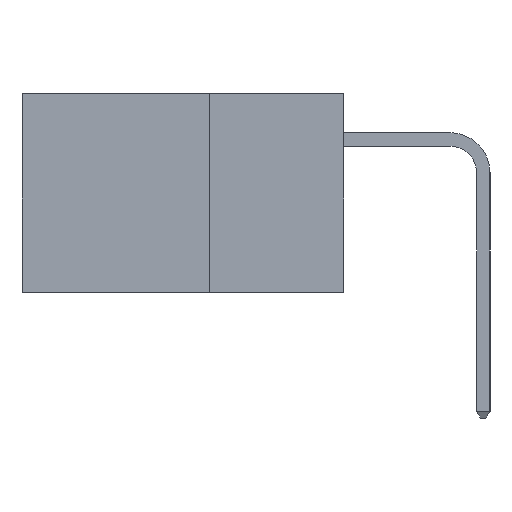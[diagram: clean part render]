
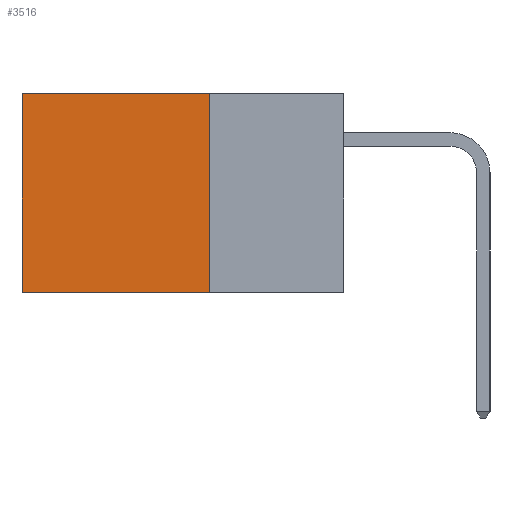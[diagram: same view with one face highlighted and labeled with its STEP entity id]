
A CAD part, left-side view. The second image highlights one B-rep face of the part: STEP entity #3516.
In plain terms, the highlighted planar face has unit normal (-1, 0, 0).
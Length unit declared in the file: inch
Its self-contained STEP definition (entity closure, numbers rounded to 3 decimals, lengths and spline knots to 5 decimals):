
#303 = CARTESIAN_POINT ( 'NONE',  ( 0.298, 0.6, -0.37 ) ) ;
#640 = CARTESIAN_POINT ( 'NONE',  ( 0.298, 0.25, 0. ) ) ;
#1190 = DIRECTION ( 'NONE',  ( 0., 0., -1. ) ) ;
#1357 = VECTOR ( 'NONE', #6439, 39.37008 ) ;
#1404 = VERTEX_POINT ( 'NONE', #2814 ) ;
#2216 = CARTESIAN_POINT ( 'NONE',  ( 0.298, 0.25, -0.37 ) ) ;
#2239 = EDGE_LOOP ( 'NONE', ( #6882, #7178, #5377, #5083 ) ) ;
#2611 = VECTOR ( 'NONE', #7909, 39.37008 ) ;
#2814 = CARTESIAN_POINT ( 'NONE',  ( 0.298, 0.6, 0. ) ) ;
#2846 = EDGE_CURVE ( 'NONE', #8374, #1404, #8167, .T. ) ;
#3516 = ADVANCED_FACE ( 'NONE', ( #6989 ), #6062, .F. ) ;
#3724 = VERTEX_POINT ( 'NONE', #3924 ) ;
#3833 = DIRECTION ( 'NONE',  ( 0., 0., -1. ) ) ;
#3924 = CARTESIAN_POINT ( 'NONE',  ( 0.298, 0.25, -0.37 ) ) ;
#5083 = ORIENTED_EDGE ( 'NONE', *, *, #2846, .T. ) ;
#5377 = ORIENTED_EDGE ( 'NONE', *, *, #9201, .F. ) ;
#5434 = AXIS2_PLACEMENT_3D ( 'NONE', #6059, #9159, #9119 ) ;
#5620 = CARTESIAN_POINT ( 'NONE',  ( 0.298, 0.25, 0. ) ) ;
#6059 = CARTESIAN_POINT ( 'NONE',  ( 0.298, 0.25, 0. ) ) ;
#6062 = PLANE ( 'NONE',  #5434 ) ;
#6166 = EDGE_CURVE ( 'NONE', #3724, #6782, #7071, .T. ) ;
#6439 = DIRECTION ( 'NONE',  ( 0., 1., 0. ) ) ;
#6532 = VECTOR ( 'NONE', #3833, 39.37008 ) ;
#6754 = LINE ( 'NONE', #7030, #6532 ) ;
#6782 = VERTEX_POINT ( 'NONE', #303 ) ;
#6825 = EDGE_CURVE ( 'NONE', #1404, #6782, #6754, .T. ) ;
#6882 = ORIENTED_EDGE ( 'NONE', *, *, #6825, .T. ) ;
#6989 = FACE_OUTER_BOUND ( 'NONE', #2239, .T. ) ;
#7030 = CARTESIAN_POINT ( 'NONE',  ( 0.298, 0.6, 0. ) ) ;
#7071 = LINE ( 'NONE', #2216, #1357 ) ;
#7178 = ORIENTED_EDGE ( 'NONE', *, *, #6166, .F. ) ;
#7909 = DIRECTION ( 'NONE',  ( 0., 1., 0. ) ) ;
#7967 = VECTOR ( 'NONE', #1190, 39.37008 ) ;
#8167 = LINE ( 'NONE', #640, #2611 ) ;
#8172 = LINE ( 'NONE', #5620, #7967 ) ;
#8374 = VERTEX_POINT ( 'NONE', #8658 ) ;
#8658 = CARTESIAN_POINT ( 'NONE',  ( 0.298, 0.25, 0. ) ) ;
#9119 = DIRECTION ( 'NONE',  ( 0., 0., -1. ) ) ;
#9159 = DIRECTION ( 'NONE',  ( 1., 0., 0. ) ) ;
#9201 = EDGE_CURVE ( 'NONE', #8374, #3724, #8172, .T. ) ;
